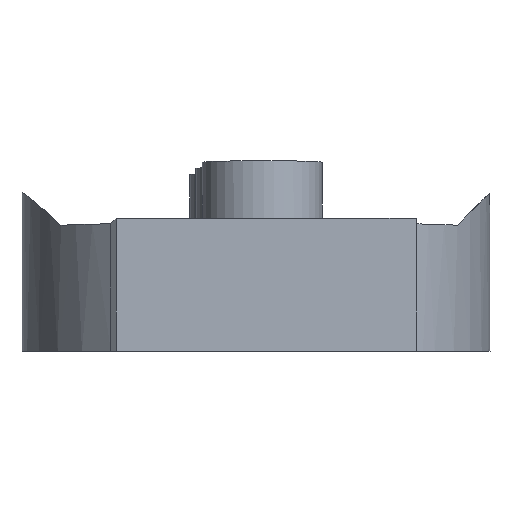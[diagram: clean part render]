
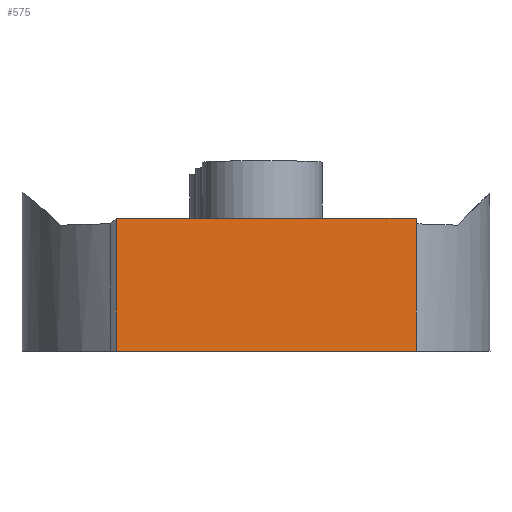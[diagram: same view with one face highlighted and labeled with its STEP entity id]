
A CAD part, left-side view. The second image highlights one B-rep face of the part: STEP entity #575.
In plain terms, the highlighted planar face has unit normal (-0.999, -0.026, 0.026).
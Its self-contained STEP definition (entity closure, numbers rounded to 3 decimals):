
#3 = CARTESIAN_POINT ( 'NONE',  ( 68.001, -25.686, 0. ) ) ;
#5 = VERTEX_POINT ( 'NONE', #288 ) ;
#57 = EDGE_CURVE ( 'NONE', #158, #394, #600, .T. ) ;
#144 = ORIENTED_EDGE ( 'NONE', *, *, #603, .F. ) ;
#157 = DIRECTION ( 'NONE',  ( -0.026, -0.001, -1. ) ) ;
#158 = VERTEX_POINT ( 'NONE', #280 ) ;
#166 = ORIENTED_EDGE ( 'NONE', *, *, #357, .F. ) ;
#171 = VECTOR ( 'NONE', #436, 1000. ) ;
#173 = ORIENTED_EDGE ( 'NONE', *, *, #57, .T. ) ;
#185 = LINE ( 'NONE', #586, #281 ) ;
#228 = DIRECTION ( 'NONE',  ( -0.026, -0.001, -1. ) ) ;
#235 = DIRECTION ( 'NONE',  ( 0.026, -1., 0. ) ) ;
#238 = FACE_OUTER_BOUND ( 'NONE', #668, .T. ) ;
#274 = CARTESIAN_POINT ( 'NONE',  ( 70.012, -19.281, 82.815 ) ) ;
#280 = CARTESIAN_POINT ( 'NONE',  ( 67.815, -12.987, 5.625 ) ) ;
#281 = VECTOR ( 'NONE', #228, 1000. ) ;
#288 = CARTESIAN_POINT ( 'NONE',  ( 68.149, -25.683, 5.625 ) ) ;
#290 = CARTESIAN_POINT ( 'NONE',  ( 68.202, -27.727, 5.625 ) ) ;
#314 = DIRECTION ( 'NONE',  ( 0.999, 0.026, -0.026 ) ) ;
#327 = LINE ( 'NONE', #433, #171 ) ;
#357 = EDGE_CURVE ( 'NONE', #5, #640, #185, .T. ) ;
#369 = VECTOR ( 'NONE', #157, 1000. ) ;
#394 = VERTEX_POINT ( 'NONE', #462 ) ;
#404 = AXIS2_PLACEMENT_3D ( 'NONE', #274, #314, #661 ) ;
#410 = CARTESIAN_POINT ( 'NONE',  ( 69.845, -12.934, 82.815 ) ) ;
#433 = CARTESIAN_POINT ( 'NONE',  ( 67.473, -5.627, 0. ) ) ;
#436 = DIRECTION ( 'NONE',  ( -0.026, 1., 0. ) ) ;
#462 = CARTESIAN_POINT ( 'NONE',  ( 67.667, -12.991, 0. ) ) ;
#510 = PLANE ( 'NONE',  #404 ) ;
#523 = LINE ( 'NONE', #290, #647 ) ;
#528 = EDGE_CURVE ( 'NONE', #640, #394, #327, .T. ) ;
#575 = ADVANCED_FACE ( 'NONE', ( #238 ), #510, .F. ) ;
#586 = CARTESIAN_POINT ( 'NONE',  ( 70.179, -25.629, 82.815 ) ) ;
#600 = LINE ( 'NONE', #410, #369 ) ;
#603 = EDGE_CURVE ( 'NONE', #158, #5, #523, .T. ) ;
#633 = ORIENTED_EDGE ( 'NONE', *, *, #528, .F. ) ;
#640 = VERTEX_POINT ( 'NONE', #3 ) ;
#647 = VECTOR ( 'NONE', #235, 1000. ) ;
#661 = DIRECTION ( 'NONE',  ( -0.026, 1., 0. ) ) ;
#668 = EDGE_LOOP ( 'NONE', ( #173, #633, #166, #144 ) ) ;
